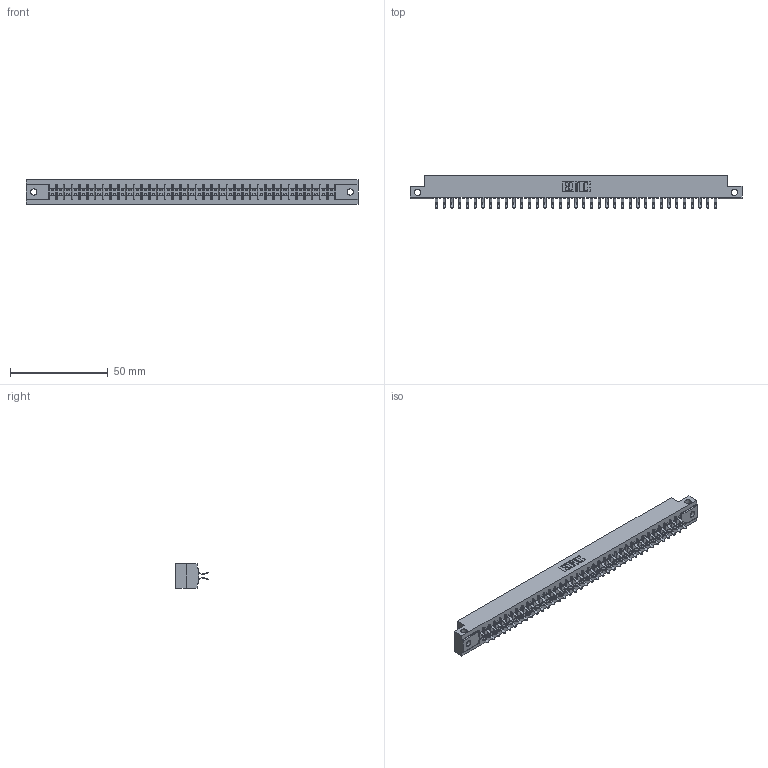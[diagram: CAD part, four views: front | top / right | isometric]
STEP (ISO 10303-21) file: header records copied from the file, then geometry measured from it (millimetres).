
FILE_DESCRIPTION (( 'STEP AP203' ), '1' );
FILE_NAME ('305-074-556-512.STEP', '2020-09-20T00:36:43', ( '' ), ( '' ), 'SwSTEP 2.0', 'SolidWorks 2020', '' );
FILE_SCHEMA (( 'CONFIG_CONTROL_DESIGN' ));
Length unit declared in the file: inch
Products named in the file (3): 305 Part_.128 Dia; 305-074-556-512; 305-290-001_556
Assembly tree (75 placements, depth 2):
  305-074-556-512
    305 Part_.128 Dia
    305-290-001_556  x74
Bounding box: 169.62 x 16.64 x 12.7 mm (x, y, z)
Volume: 16941 mm3; surface area: 22362.3 mm2
Topology: 75 solids, 75 shells, 4272 faces, 12303 edges, 7998 vertices
Faces by surface type: plane 2362, cylinder 1762, sphere 148
Entity records: 41298 total; most frequent: CARTESIAN_POINT 6885, ORIENTED_EDGE 6790, DIRECTION 6607, EDGE_CURVE 3395, VECTOR 2719, LINE 2719, VERTEX_POINT 2158, AXIS2_PLACEMENT_3D 1944
